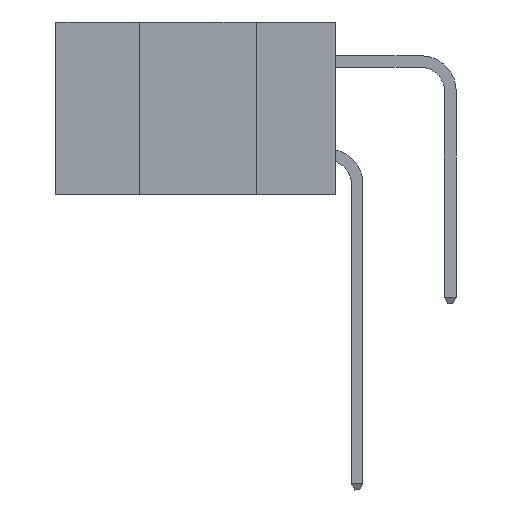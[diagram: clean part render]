
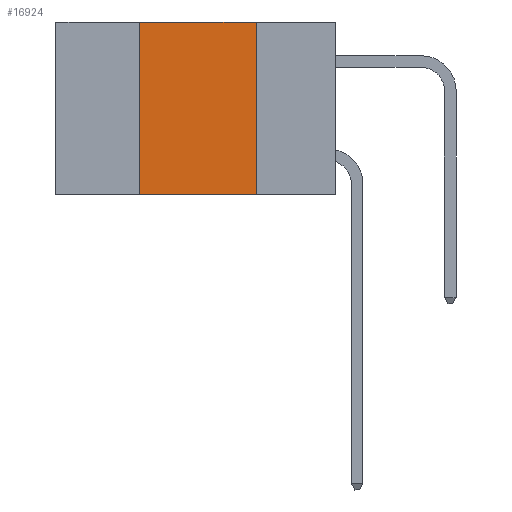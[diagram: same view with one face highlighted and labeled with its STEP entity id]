
A CAD part, left-side view. The second image highlights one B-rep face of the part: STEP entity #16924.
In plain terms, the highlighted planar face has unit normal (-1, 0, 0).
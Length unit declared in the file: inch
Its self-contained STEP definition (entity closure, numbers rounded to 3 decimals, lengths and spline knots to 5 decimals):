
#260 = CARTESIAN_POINT ( 'NONE',  ( 0., 0.17, -0.37 ) ) ;
#1164 = CARTESIAN_POINT ( 'NONE',  ( 0., 0.17, 0. ) ) ;
#3375 = AXIS2_PLACEMENT_3D ( 'NONE', #25698, #25343, #9675 ) ;
#7127 = DIRECTION ( 'NONE',  ( 0., 0., -1. ) ) ;
#8007 = VECTOR ( 'NONE', #7127, 39.37008 ) ;
#9494 = PLANE ( 'NONE',  #3375 ) ;
#9671 = VECTOR ( 'NONE', #32036, 39.37008 ) ;
#9675 = DIRECTION ( 'NONE',  ( 0., 0., -1. ) ) ;
#10123 = ORIENTED_EDGE ( 'NONE', *, *, #18980, .T. ) ;
#11744 = VECTOR ( 'NONE', #12846, 39.37008 ) ;
#12549 = ORIENTED_EDGE ( 'NONE', *, *, #20742, .F. ) ;
#12846 = DIRECTION ( 'NONE',  ( 0., 0., 1. ) ) ;
#13012 = ORIENTED_EDGE ( 'NONE', *, *, #34255, .F. ) ;
#13163 = CARTESIAN_POINT ( 'NONE',  ( 0., 0.6, -0.37 ) ) ;
#14341 = EDGE_CURVE ( 'NONE', #21149, #25438, #23326, .T. ) ;
#15290 = LINE ( 'NONE', #13163, #9671 ) ;
#16581 = VECTOR ( 'NONE', #24598, 39.37008 ) ;
#16786 = EDGE_LOOP ( 'NONE', ( #21299, #12549, #13012, #10123 ) ) ;
#16924 = ADVANCED_FACE ( 'NONE', ( #20531 ), #9494, .F. ) ;
#17831 = LINE ( 'NONE', #29229, #11744 ) ;
#18564 = VERTEX_POINT ( 'NONE', #31409 ) ;
#18980 = EDGE_CURVE ( 'NONE', #34945, #25438, #15290, .T. ) ;
#20531 = FACE_OUTER_BOUND ( 'NONE', #16786, .T. ) ;
#20742 = EDGE_CURVE ( 'NONE', #18564, #21149, #27272, .T. ) ;
#21149 = VERTEX_POINT ( 'NONE', #1164 ) ;
#21165 = CARTESIAN_POINT ( 'NONE',  ( 0., 0.42, -0.37 ) ) ;
#21299 = ORIENTED_EDGE ( 'NONE', *, *, #14341, .F. ) ;
#23326 = LINE ( 'NONE', #28307, #8007 ) ;
#24598 = DIRECTION ( 'NONE',  ( 0., -1., 0. ) ) ;
#25343 = DIRECTION ( 'NONE',  ( 1., 0., 0. ) ) ;
#25438 = VERTEX_POINT ( 'NONE', #260 ) ;
#25698 = CARTESIAN_POINT ( 'NONE',  ( 0., 0.6, 0. ) ) ;
#27272 = LINE ( 'NONE', #32782, #16581 ) ;
#28307 = CARTESIAN_POINT ( 'NONE',  ( 0., 0.17, 0. ) ) ;
#29229 = CARTESIAN_POINT ( 'NONE',  ( 0., 0.42, 0. ) ) ;
#31409 = CARTESIAN_POINT ( 'NONE',  ( 0., 0.42, 0. ) ) ;
#32036 = DIRECTION ( 'NONE',  ( 0., -1., 0. ) ) ;
#32782 = CARTESIAN_POINT ( 'NONE',  ( 0., 0.6, 0. ) ) ;
#34255 = EDGE_CURVE ( 'NONE', #34945, #18564, #17831, .T. ) ;
#34945 = VERTEX_POINT ( 'NONE', #21165 ) ;
